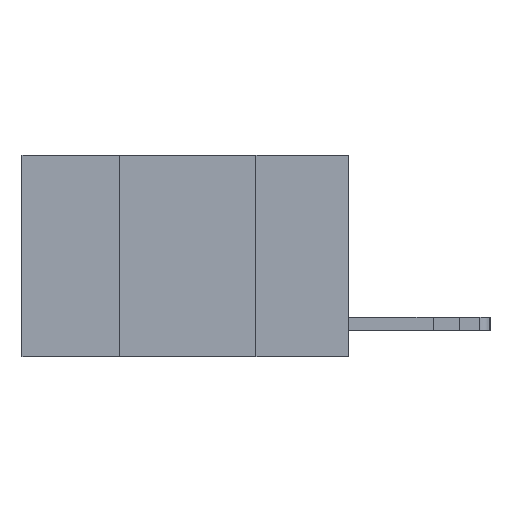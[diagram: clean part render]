
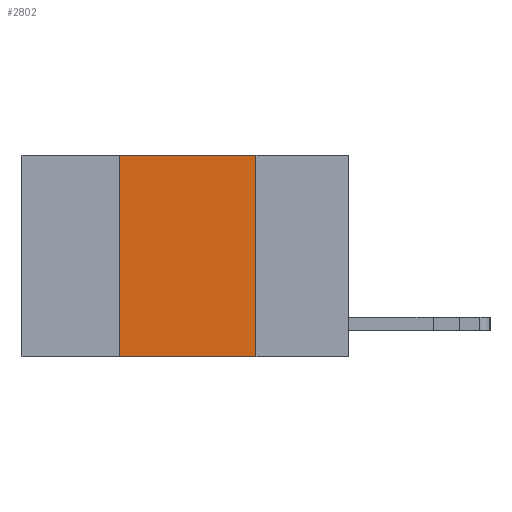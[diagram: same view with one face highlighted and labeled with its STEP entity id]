
A CAD part, left-side view. The second image highlights one B-rep face of the part: STEP entity #2802.
In plain terms, the highlighted planar face has unit normal (-1, 0, 0).
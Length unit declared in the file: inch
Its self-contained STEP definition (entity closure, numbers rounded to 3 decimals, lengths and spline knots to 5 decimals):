
#313 = VERTEX_POINT ( 'NONE', #4983 ) ;
#558 = ORIENTED_EDGE ( 'NONE', *, *, #7022, .F. ) ;
#575 = VERTEX_POINT ( 'NONE', #5095 ) ;
#825 = VECTOR ( 'NONE', #6452, 39.37008 ) ;
#1120 = LINE ( 'NONE', #10856, #825 ) ;
#1418 = CARTESIAN_POINT ( 'NONE',  ( 0., 0.42, 0. ) ) ;
#1722 = VECTOR ( 'NONE', #2714, 39.37008 ) ;
#2564 = ORIENTED_EDGE ( 'NONE', *, *, #9140, .T. ) ;
#2714 = DIRECTION ( 'NONE',  ( 0., -1., 0. ) ) ;
#2802 = ADVANCED_FACE ( 'NONE', ( #7423 ), #8124, .F. ) ;
#3412 = EDGE_LOOP ( 'NONE', ( #9619, #558, #11568, #2564 ) ) ;
#3506 = CARTESIAN_POINT ( 'NONE',  ( 0., 0.6, 0. ) ) ;
#3681 = VECTOR ( 'NONE', #4150, 39.37008 ) ;
#3935 = CARTESIAN_POINT ( 'NONE',  ( 0., 0.6, -0.37 ) ) ;
#4150 = DIRECTION ( 'NONE',  ( 0., 0., 1. ) ) ;
#4796 = DIRECTION ( 'NONE',  ( 1., 0., 0. ) ) ;
#4804 = DIRECTION ( 'NONE',  ( 0., -1., 0. ) ) ;
#4983 = CARTESIAN_POINT ( 'NONE',  ( 0., 0.42, -0.37 ) ) ;
#5095 = CARTESIAN_POINT ( 'NONE',  ( 0., 0.42, 0. ) ) ;
#5631 = VECTOR ( 'NONE', #4804, 39.37008 ) ;
#5672 = VERTEX_POINT ( 'NONE', #9078 ) ;
#6312 = LINE ( 'NONE', #1418, #3681 ) ;
#6452 = DIRECTION ( 'NONE',  ( 0., 0., -1. ) ) ;
#6457 = AXIS2_PLACEMENT_3D ( 'NONE', #3506, #4796, #6618 ) ;
#6480 = LINE ( 'NONE', #8908, #1722 ) ;
#6618 = DIRECTION ( 'NONE',  ( 0., 0., -1. ) ) ;
#7022 = EDGE_CURVE ( 'NONE', #575, #8378, #6480, .T. ) ;
#7423 = FACE_OUTER_BOUND ( 'NONE', #3412, .T. ) ;
#8121 = EDGE_CURVE ( 'NONE', #313, #575, #6312, .T. ) ;
#8124 = PLANE ( 'NONE',  #6457 ) ;
#8378 = VERTEX_POINT ( 'NONE', #8996 ) ;
#8435 = EDGE_CURVE ( 'NONE', #8378, #5672, #1120, .T. ) ;
#8908 = CARTESIAN_POINT ( 'NONE',  ( 0., 0.6, 0. ) ) ;
#8996 = CARTESIAN_POINT ( 'NONE',  ( 0., 0.17, 0. ) ) ;
#9078 = CARTESIAN_POINT ( 'NONE',  ( 0., 0.17, -0.37 ) ) ;
#9140 = EDGE_CURVE ( 'NONE', #313, #5672, #10027, .T. ) ;
#9619 = ORIENTED_EDGE ( 'NONE', *, *, #8435, .F. ) ;
#10027 = LINE ( 'NONE', #3935, #5631 ) ;
#10856 = CARTESIAN_POINT ( 'NONE',  ( 0., 0.17, 0. ) ) ;
#11568 = ORIENTED_EDGE ( 'NONE', *, *, #8121, .F. ) ;
